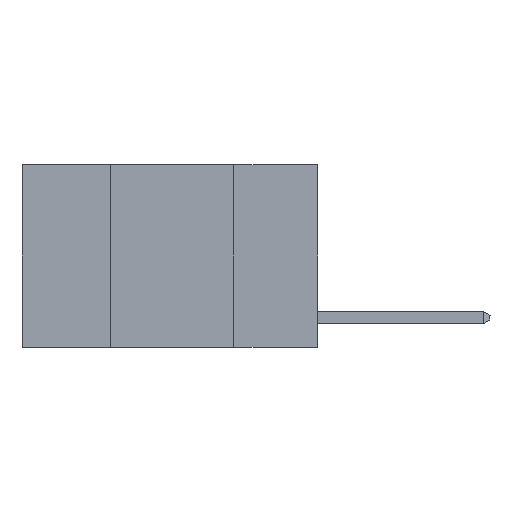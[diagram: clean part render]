
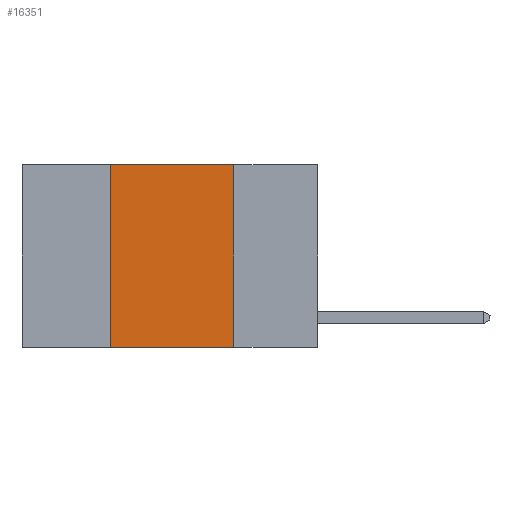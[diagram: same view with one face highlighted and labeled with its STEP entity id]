
A CAD part, left-side view. The second image highlights one B-rep face of the part: STEP entity #16351.
In plain terms, the highlighted planar face has unit normal (-1, 0, 0).
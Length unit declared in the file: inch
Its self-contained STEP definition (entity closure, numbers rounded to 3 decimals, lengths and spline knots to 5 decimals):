
#850 = CARTESIAN_POINT ( 'NONE',  ( 0., 0.42, 0. ) ) ;
#1611 = EDGE_CURVE ( 'NONE', #23395, #7363, #2413, .T. ) ;
#1749 = DIRECTION ( 'NONE',  ( 0., 0., -1. ) ) ;
#2413 = LINE ( 'NONE', #11146, #21162 ) ;
#2485 = CARTESIAN_POINT ( 'NONE',  ( 0., 0.17, 0. ) ) ;
#3061 = VECTOR ( 'NONE', #13706, 39.37008 ) ;
#3207 = EDGE_CURVE ( 'NONE', #17383, #20067, #9647, .T. ) ;
#3961 = CARTESIAN_POINT ( 'NONE',  ( 0., 0.42, -0.37 ) ) ;
#4970 = CARTESIAN_POINT ( 'NONE',  ( 0., 0.17, -0.37 ) ) ;
#5012 = DIRECTION ( 'NONE',  ( 0., -1., 0. ) ) ;
#7159 = EDGE_CURVE ( 'NONE', #20067, #7363, #12977, .T. ) ;
#7363 = VERTEX_POINT ( 'NONE', #4970 ) ;
#7758 = DIRECTION ( 'NONE',  ( 0., -1., 0. ) ) ;
#8511 = CARTESIAN_POINT ( 'NONE',  ( 0., 0.42, 0. ) ) ;
#9414 = ORIENTED_EDGE ( 'NONE', *, *, #1611, .T. ) ;
#9647 = LINE ( 'NONE', #18036, #14020 ) ;
#10289 = AXIS2_PLACEMENT_3D ( 'NONE', #11085, #12973, #1749 ) ;
#11085 = CARTESIAN_POINT ( 'NONE',  ( 0., 0.6, 0. ) ) ;
#11146 = CARTESIAN_POINT ( 'NONE',  ( 0., 0.6, -0.37 ) ) ;
#12973 = DIRECTION ( 'NONE',  ( 1., 0., 0. ) ) ;
#12977 = LINE ( 'NONE', #2485, #3061 ) ;
#13209 = ORIENTED_EDGE ( 'NONE', *, *, #3207, .F. ) ;
#13706 = DIRECTION ( 'NONE',  ( 0., 0., -1. ) ) ;
#14020 = VECTOR ( 'NONE', #5012, 39.37008 ) ;
#14231 = FACE_OUTER_BOUND ( 'NONE', #23027, .T. ) ;
#14350 = LINE ( 'NONE', #8511, #24275 ) ;
#16351 = ADVANCED_FACE ( 'NONE', ( #14231 ), #24149, .F. ) ;
#16973 = ORIENTED_EDGE ( 'NONE', *, *, #7159, .F. ) ;
#17383 = VERTEX_POINT ( 'NONE', #850 ) ;
#17883 = CARTESIAN_POINT ( 'NONE',  ( 0., 0.17, 0. ) ) ;
#18036 = CARTESIAN_POINT ( 'NONE',  ( 0., 0.6, 0. ) ) ;
#19658 = EDGE_CURVE ( 'NONE', #23395, #17383, #14350, .T. ) ;
#20067 = VERTEX_POINT ( 'NONE', #17883 ) ;
#21162 = VECTOR ( 'NONE', #7758, 39.37008 ) ;
#21578 = DIRECTION ( 'NONE',  ( 0., 0., 1. ) ) ;
#21995 = ORIENTED_EDGE ( 'NONE', *, *, #19658, .F. ) ;
#23027 = EDGE_LOOP ( 'NONE', ( #16973, #13209, #21995, #9414 ) ) ;
#23395 = VERTEX_POINT ( 'NONE', #3961 ) ;
#24149 = PLANE ( 'NONE',  #10289 ) ;
#24275 = VECTOR ( 'NONE', #21578, 39.37008 ) ;
